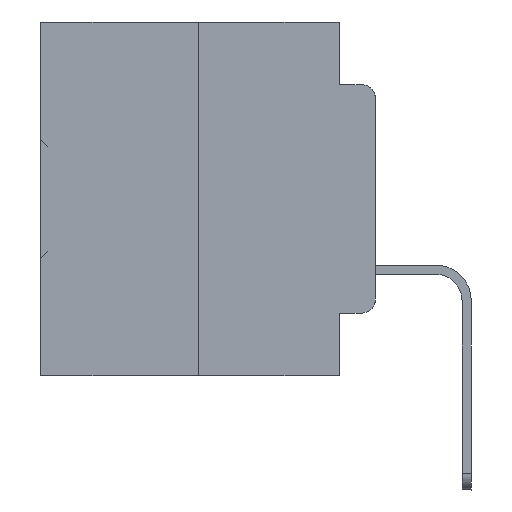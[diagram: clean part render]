
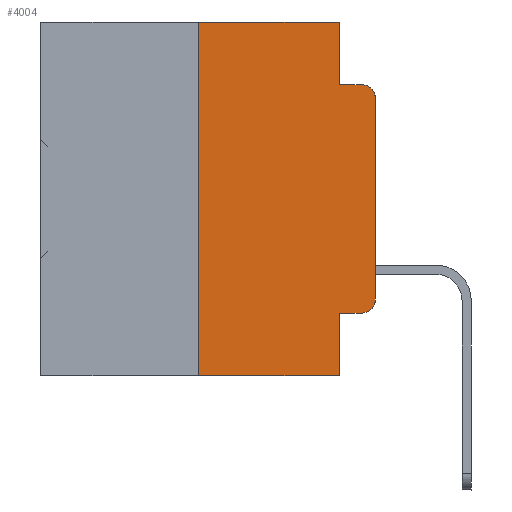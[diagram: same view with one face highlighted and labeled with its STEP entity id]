
A CAD part, left-side view. The second image highlights one B-rep face of the part: STEP entity #4004.
In plain terms, the highlighted planar face has unit normal (-1, 0, 0).
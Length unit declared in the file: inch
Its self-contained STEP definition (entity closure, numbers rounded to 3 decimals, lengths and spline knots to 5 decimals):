
#166 = VERTEX_POINT ( 'NONE', #22530 ) ;
#489 = LINE ( 'NONE', #32375, #7323 ) ;
#522 = PLANE ( 'NONE',  #28069 ) ;
#1143 = VERTEX_POINT ( 'NONE', #13489 ) ;
#1233 = CARTESIAN_POINT ( 'NONE',  ( 0., 0.051, 0. ) ) ;
#1250 = CARTESIAN_POINT ( 'NONE',  ( 0., 0.02, -0.3915 ) ) ;
#2674 = ORIENTED_EDGE ( 'NONE', *, *, #25900, .T. ) ;
#2838 = CARTESIAN_POINT ( 'NONE',  ( 0., 0.473, 0. ) ) ;
#3130 = VERTEX_POINT ( 'NONE', #24517 ) ;
#3154 = DIRECTION ( 'NONE',  ( 0., -1., 0. ) ) ;
#3502 = EDGE_CURVE ( 'NONE', #1143, #20373, #7473, .T. ) ;
#3784 = CARTESIAN_POINT ( 'NONE',  ( 0., 0.051, -0.4115 ) ) ;
#3818 = ORIENTED_EDGE ( 'NONE', *, *, #25807, .T. ) ;
#4004 = ADVANCED_FACE ( 'NONE', ( #17557 ), #522, .F. ) ;
#4908 = VECTOR ( 'NONE', #6725, 39.37008 ) ;
#5096 = EDGE_CURVE ( 'NONE', #32539, #37572, #36777, .T. ) ;
#6702 = VECTOR ( 'NONE', #19048, 39.37008 ) ;
#6725 = DIRECTION ( 'NONE',  ( 0., -1., 0. ) ) ;
#6884 = CIRCLE ( 'NONE', #7660, 0.02 ) ;
#7323 = VECTOR ( 'NONE', #3154, 39.37008 ) ;
#7473 = LINE ( 'NONE', #2838, #29040 ) ;
#7660 = AXIS2_PLACEMENT_3D ( 'NONE', #1250, #33549, #36774 ) ;
#8834 = DIRECTION ( 'NONE',  ( -1., 0., 0. ) ) ;
#10690 = EDGE_CURVE ( 'NONE', #31834, #1143, #14271, .T. ) ;
#11114 = CARTESIAN_POINT ( 'NONE',  ( 0., 0.051, -0.0885 ) ) ;
#12017 = DIRECTION ( 'NONE',  ( 1., 0., 0. ) ) ;
#13489 = CARTESIAN_POINT ( 'NONE',  ( 0., 0.25, 0. ) ) ;
#14070 = ORIENTED_EDGE ( 'NONE', *, *, #15417, .T. ) ;
#14271 = LINE ( 'NONE', #23830, #27550 ) ;
#15248 = DIRECTION ( 'NONE',  ( 0., 0., 1. ) ) ;
#15417 = EDGE_CURVE ( 'NONE', #31834, #23688, #489, .T. ) ;
#15529 = DIRECTION ( 'NONE',  ( 0., 0., -1. ) ) ;
#15700 = EDGE_LOOP ( 'NONE', ( #2674, #28783, #18958, #29743, #32434, #21693, #14070, #19372, #33806, #3818 ) ) ;
#16599 = CARTESIAN_POINT ( 'NONE',  ( 0., 0.051, -0.5 ) ) ;
#17270 = EDGE_CURVE ( 'NONE', #20373, #32539, #35669, .T. ) ;
#17557 = FACE_OUTER_BOUND ( 'NONE', #15700, .T. ) ;
#18132 = CIRCLE ( 'NONE', #26639, 0.02 ) ;
#18220 = EDGE_CURVE ( 'NONE', #33849, #37572, #18132, .T. ) ;
#18228 = EDGE_CURVE ( 'NONE', #166, #23688, #36038, .T. ) ;
#18725 = CARTESIAN_POINT ( 'NONE',  ( 0., 0.051, 0. ) ) ;
#18958 = ORIENTED_EDGE ( 'NONE', *, *, #5096, .F. ) ;
#19048 = DIRECTION ( 'NONE',  ( 0., 0., -1. ) ) ;
#19372 = ORIENTED_EDGE ( 'NONE', *, *, #18228, .F. ) ;
#19749 = CARTESIAN_POINT ( 'NONE',  ( 0., 0.051, 0. ) ) ;
#20373 = VERTEX_POINT ( 'NONE', #19749 ) ;
#21447 = CARTESIAN_POINT ( 'NONE',  ( 0., 0.02, -0.4115 ) ) ;
#21693 = ORIENTED_EDGE ( 'NONE', *, *, #10690, .F. ) ;
#21874 = VERTEX_POINT ( 'NONE', #21447 ) ;
#22530 = CARTESIAN_POINT ( 'NONE',  ( 0., 0.051, -0.4115 ) ) ;
#23432 = VECTOR ( 'NONE', #34627, 39.37008 ) ;
#23688 = VERTEX_POINT ( 'NONE', #16599 ) ;
#23830 = CARTESIAN_POINT ( 'NONE',  ( 0., 0.25, 0. ) ) ;
#24517 = CARTESIAN_POINT ( 'NONE',  ( 0., 0., -0.3915 ) ) ;
#25208 = DIRECTION ( 'NONE',  ( 0., 0., 1. ) ) ;
#25418 = CARTESIAN_POINT ( 'NONE',  ( 0., 0.25, -0.5 ) ) ;
#25807 = EDGE_CURVE ( 'NONE', #21874, #3130, #6884, .T. ) ;
#25900 = EDGE_CURVE ( 'NONE', #3130, #33849, #28424, .T. ) ;
#26639 = AXIS2_PLACEMENT_3D ( 'NONE', #30129, #8834, #15529 ) ;
#26769 = DIRECTION ( 'NONE',  ( 0., 0., -1. ) ) ;
#27261 = VECTOR ( 'NONE', #36188, 39.37008 ) ;
#27522 = CARTESIAN_POINT ( 'NONE',  ( 0., 0., -0.1085 ) ) ;
#27550 = VECTOR ( 'NONE', #15248, 39.37008 ) ;
#27818 = CARTESIAN_POINT ( 'NONE',  ( 0., 0.02, -0.0885 ) ) ;
#28069 = AXIS2_PLACEMENT_3D ( 'NONE', #29724, #12017, #26769 ) ;
#28297 = LINE ( 'NONE', #3784, #4908 ) ;
#28424 = LINE ( 'NONE', #31205, #30285 ) ;
#28783 = ORIENTED_EDGE ( 'NONE', *, *, #18220, .T. ) ;
#29040 = VECTOR ( 'NONE', #35827, 39.37008 ) ;
#29406 = EDGE_CURVE ( 'NONE', #166, #21874, #28297, .T. ) ;
#29724 = CARTESIAN_POINT ( 'NONE',  ( 0., 0.473, 0. ) ) ;
#29743 = ORIENTED_EDGE ( 'NONE', *, *, #17270, .F. ) ;
#30129 = CARTESIAN_POINT ( 'NONE',  ( 0., 0.02, -0.1085 ) ) ;
#30285 = VECTOR ( 'NONE', #25208, 39.37008 ) ;
#30631 = CARTESIAN_POINT ( 'NONE',  ( 0., 0.051, -0.0885 ) ) ;
#31205 = CARTESIAN_POINT ( 'NONE',  ( 0., 0., 0. ) ) ;
#31834 = VERTEX_POINT ( 'NONE', #25418 ) ;
#32375 = CARTESIAN_POINT ( 'NONE',  ( 0., 0.473, -0.5 ) ) ;
#32434 = ORIENTED_EDGE ( 'NONE', *, *, #3502, .F. ) ;
#32539 = VERTEX_POINT ( 'NONE', #30631 ) ;
#33549 = DIRECTION ( 'NONE',  ( -1., 0., 0. ) ) ;
#33806 = ORIENTED_EDGE ( 'NONE', *, *, #29406, .T. ) ;
#33849 = VERTEX_POINT ( 'NONE', #27522 ) ;
#34627 = DIRECTION ( 'NONE',  ( 0., -1., 0. ) ) ;
#35669 = LINE ( 'NONE', #1233, #6702 ) ;
#35827 = DIRECTION ( 'NONE',  ( 0., -1., 0. ) ) ;
#36038 = LINE ( 'NONE', #18725, #27261 ) ;
#36188 = DIRECTION ( 'NONE',  ( 0., 0., -1. ) ) ;
#36774 = DIRECTION ( 'NONE',  ( 0., 0., -1. ) ) ;
#36777 = LINE ( 'NONE', #11114, #23432 ) ;
#37572 = VERTEX_POINT ( 'NONE', #27818 ) ;
